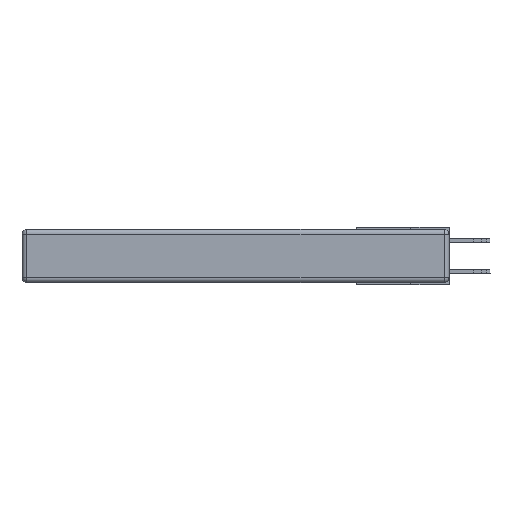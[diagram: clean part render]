
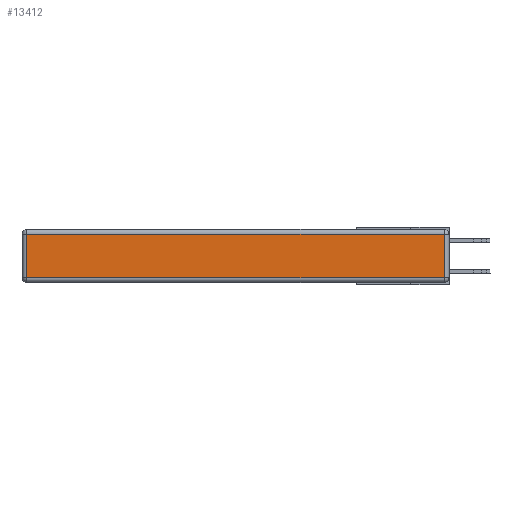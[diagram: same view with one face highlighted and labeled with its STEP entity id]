
A CAD part, left-side view. The second image highlights one B-rep face of the part: STEP entity #13412.
In plain terms, the highlighted planar face has unit normal (-1, 0, 0).
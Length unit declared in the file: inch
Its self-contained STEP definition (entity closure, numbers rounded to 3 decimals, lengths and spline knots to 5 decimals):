
#1103 = DIRECTION ( 'NONE',  ( 0., 0., -1. ) ) ;
#1177 = ORIENTED_EDGE ( 'NONE', *, *, #13214, .T. ) ;
#1772 = ORIENTED_EDGE ( 'NONE', *, *, #7161, .T. ) ;
#2503 = CARTESIAN_POINT ( 'NONE',  ( 0., 2.75, -0.03 ) ) ;
#3187 = LINE ( 'NONE', #11841, #7916 ) ;
#3452 = CARTESIAN_POINT ( 'NONE',  ( 0., 0.03, -0.313 ) ) ;
#3530 = ORIENTED_EDGE ( 'NONE', *, *, #13598, .T. ) ;
#3839 = PLANE ( 'NONE',  #12892 ) ;
#4210 = CARTESIAN_POINT ( 'NONE',  ( 0., 0., -0.313 ) ) ;
#4621 = LINE ( 'NONE', #4210, #13897 ) ;
#5263 = DIRECTION ( 'NONE',  ( 0., -1., 0. ) ) ;
#5709 = VERTEX_POINT ( 'NONE', #9583 ) ;
#5815 = VERTEX_POINT ( 'NONE', #11836 ) ;
#5875 = VERTEX_POINT ( 'NONE', #7397 ) ;
#5986 = EDGE_CURVE ( 'NONE', #5815, #5709, #11328, .T. ) ;
#6103 = DIRECTION ( 'NONE',  ( -1., 0., 0. ) ) ;
#7161 = EDGE_CURVE ( 'NONE', #10931, #5875, #3187, .T. ) ;
#7397 = CARTESIAN_POINT ( 'NONE',  ( 0., 0.03, -0.03 ) ) ;
#7547 = DIRECTION ( 'NONE',  ( 0., 0., 1. ) ) ;
#7916 = VECTOR ( 'NONE', #7547, 39.37008 ) ;
#8143 = CARTESIAN_POINT ( 'NONE',  ( 0., 0., -0.343 ) ) ;
#8446 = ORIENTED_EDGE ( 'NONE', *, *, #5986, .T. ) ;
#9323 = DIRECTION ( 'NONE',  ( 0., 0., 1. ) ) ;
#9538 = EDGE_LOOP ( 'NONE', ( #3530, #1772, #1177, #8446 ) ) ;
#9583 = CARTESIAN_POINT ( 'NONE',  ( 0., 2.72, -0.313 ) ) ;
#9619 = CARTESIAN_POINT ( 'NONE',  ( 0., 2.72, -0.343 ) ) ;
#10375 = FACE_OUTER_BOUND ( 'NONE', #9538, .T. ) ;
#10728 = LINE ( 'NONE', #2503, #11083 ) ;
#10931 = VERTEX_POINT ( 'NONE', #3452 ) ;
#11083 = VECTOR ( 'NONE', #11175, 39.37008 ) ;
#11175 = DIRECTION ( 'NONE',  ( 0., 1., 0. ) ) ;
#11328 = LINE ( 'NONE', #9619, #13826 ) ;
#11836 = CARTESIAN_POINT ( 'NONE',  ( 0., 2.72, -0.03 ) ) ;
#11841 = CARTESIAN_POINT ( 'NONE',  ( 0., 0.03, -0.343 ) ) ;
#12892 = AXIS2_PLACEMENT_3D ( 'NONE', #8143, #6103, #9323 ) ;
#13214 = EDGE_CURVE ( 'NONE', #5875, #5815, #10728, .T. ) ;
#13412 = ADVANCED_FACE ( 'NONE', ( #10375 ), #3839, .T. ) ;
#13598 = EDGE_CURVE ( 'NONE', #5709, #10931, #4621, .T. ) ;
#13826 = VECTOR ( 'NONE', #1103, 39.37008 ) ;
#13897 = VECTOR ( 'NONE', #5263, 39.37008 ) ;
